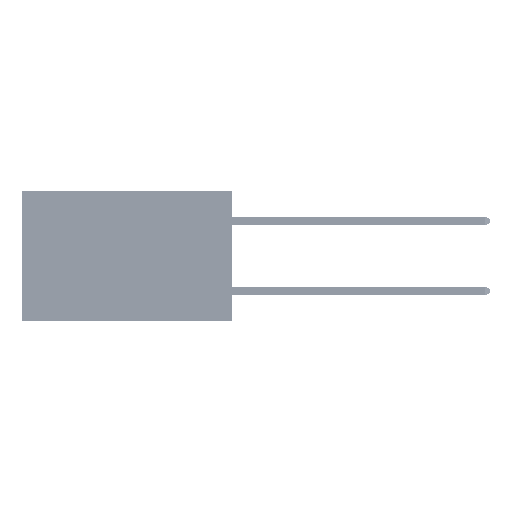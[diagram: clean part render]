
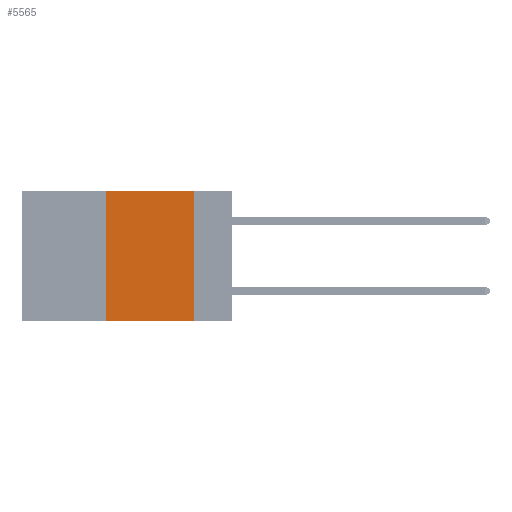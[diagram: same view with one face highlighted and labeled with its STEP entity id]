
A CAD part, left-side view. The second image highlights one B-rep face of the part: STEP entity #5565.
In plain terms, the highlighted planar face has unit normal (-1, 0, 0).
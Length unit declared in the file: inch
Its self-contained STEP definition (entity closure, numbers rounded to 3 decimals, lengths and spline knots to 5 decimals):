
#5565 = ADVANCED_FACE ( 'NONE', ( #10713 ), #8807, .F. ) ;
#8807 = PLANE ( 'NONE',  #39497 ) ;
#10713 = FACE_OUTER_BOUND ( 'NONE', #17851, .T. ) ;
#12638 = VECTOR ( 'NONE', #19556, 39.37008 ) ;
#13157 = DIRECTION ( 'NONE',  ( 0., 0., -1. ) ) ;
#13421 = ORIENTED_EDGE ( 'NONE', *, *, #26770, .F. ) ;
#14325 = VECTOR ( 'NONE', #20609, 39.37008 ) ;
#15048 = LINE ( 'NONE', #23562, #12638 ) ;
#17851 = EDGE_LOOP ( 'NONE', ( #33625, #13421, #18444, #20100 ) ) ;
#18444 = ORIENTED_EDGE ( 'NONE', *, *, #33166, .F. ) ;
#19556 = DIRECTION ( 'NONE',  ( 0., -1., 0. ) ) ;
#20100 = ORIENTED_EDGE ( 'NONE', *, *, #44863, .T. ) ;
#20526 = CARTESIAN_POINT ( 'NONE',  ( 0., 0.36, 0. ) ) ;
#20609 = DIRECTION ( 'NONE',  ( 0., -1., 0. ) ) ;
#21135 = VECTOR ( 'NONE', #47936, 39.37008 ) ;
#21765 = VERTEX_POINT ( 'NONE', #27595 ) ;
#22183 = DIRECTION ( 'NONE',  ( 0., 0., -1. ) ) ;
#23562 = CARTESIAN_POINT ( 'NONE',  ( 0., 0.6, 0. ) ) ;
#26770 = EDGE_CURVE ( 'NONE', #31694, #21765, #15048, .T. ) ;
#27595 = CARTESIAN_POINT ( 'NONE',  ( 0., 0.11, 0. ) ) ;
#28223 = LINE ( 'NONE', #28369, #14325 ) ;
#28369 = CARTESIAN_POINT ( 'NONE',  ( 0., 0.6, -0.37 ) ) ;
#31694 = VERTEX_POINT ( 'NONE', #20526 ) ;
#32002 = LINE ( 'NONE', #48272, #21135 ) ;
#33166 = EDGE_CURVE ( 'NONE', #38499, #31694, #32002, .T. ) ;
#33625 = ORIENTED_EDGE ( 'NONE', *, *, #37068, .F. ) ;
#36202 = DIRECTION ( 'NONE',  ( 1., 0., 0. ) ) ;
#36867 = CARTESIAN_POINT ( 'NONE',  ( 0., 0.11, -0.37 ) ) ;
#36910 = LINE ( 'NONE', #45302, #41122 ) ;
#37068 = EDGE_CURVE ( 'NONE', #21765, #43321, #36910, .T. ) ;
#38499 = VERTEX_POINT ( 'NONE', #48246 ) ;
#39497 = AXIS2_PLACEMENT_3D ( 'NONE', #47356, #36202, #13157 ) ;
#41122 = VECTOR ( 'NONE', #22183, 39.37008 ) ;
#43321 = VERTEX_POINT ( 'NONE', #36867 ) ;
#44863 = EDGE_CURVE ( 'NONE', #38499, #43321, #28223, .T. ) ;
#45302 = CARTESIAN_POINT ( 'NONE',  ( 0., 0.11, 0. ) ) ;
#47356 = CARTESIAN_POINT ( 'NONE',  ( 0., 0.6, 0. ) ) ;
#47936 = DIRECTION ( 'NONE',  ( 0., 0., 1. ) ) ;
#48246 = CARTESIAN_POINT ( 'NONE',  ( 0., 0.36, -0.37 ) ) ;
#48272 = CARTESIAN_POINT ( 'NONE',  ( 0., 0.36, 0. ) ) ;
